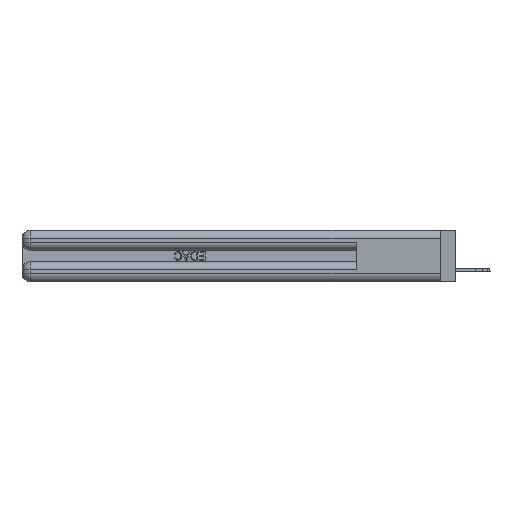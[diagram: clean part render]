
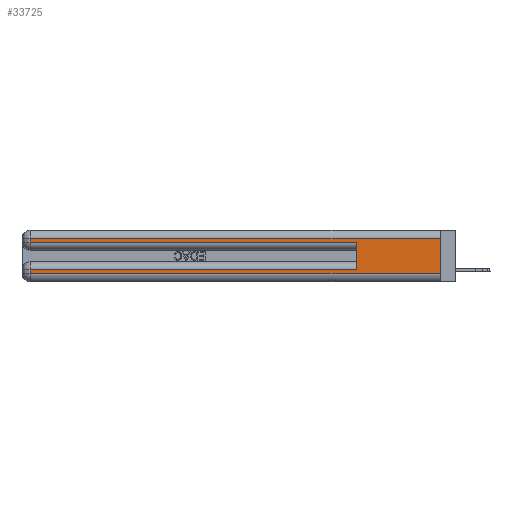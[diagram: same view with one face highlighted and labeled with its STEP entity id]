
A CAD part, left-side view. The second image highlights one B-rep face of the part: STEP entity #33725.
In plain terms, the highlighted planar face has unit normal (-1, 0, 0).
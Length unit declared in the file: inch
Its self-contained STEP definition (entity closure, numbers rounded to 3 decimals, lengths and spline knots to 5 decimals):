
#102 = DIRECTION ( 'NONE',  ( 0., -1., 0. ) ) ;
#220 = CARTESIAN_POINT ( 'NONE',  ( 0., 0., 0.285 ) ) ;
#392 = LINE ( 'NONE', #25619, #35999 ) ;
#620 = DIRECTION ( 'NONE',  ( 0., 1., 0. ) ) ;
#663 = EDGE_CURVE ( 'NONE', #34133, #27485, #3351, .T. ) ;
#842 = DIRECTION ( 'NONE',  ( 0., 0., -1. ) ) ;
#1767 = CARTESIAN_POINT ( 'NONE',  ( 0., 2.94, 0.285 ) ) ;
#1819 = CARTESIAN_POINT ( 'NONE',  ( 0., 0.6, 0.145 ) ) ;
#3016 = VERTEX_POINT ( 'NONE', #15526 ) ;
#3038 = VECTOR ( 'NONE', #6035, 39.37008 ) ;
#3351 = LINE ( 'NONE', #220, #6422 ) ;
#3595 = EDGE_CURVE ( 'NONE', #3016, #16636, #392, .T. ) ;
#4185 = LINE ( 'NONE', #19852, #24195 ) ;
#4633 = EDGE_LOOP ( 'NONE', ( #14149, #35008, #35609, #28040, #35874, #6933, #33448, #26361 ) ) ;
#5358 = AXIS2_PLACEMENT_3D ( 'NONE', #8840, #5862, #34517 ) ;
#5862 = DIRECTION ( 'NONE',  ( 1., 0., 0. ) ) ;
#6035 = DIRECTION ( 'NONE',  ( 0., 1., 0. ) ) ;
#6422 = VECTOR ( 'NONE', #20336, 39.37008 ) ;
#6619 = EDGE_CURVE ( 'NONE', #3016, #26334, #10309, .T. ) ;
#6933 = ORIENTED_EDGE ( 'NONE', *, *, #26800, .T. ) ;
#7056 = CARTESIAN_POINT ( 'NONE',  ( 0., 2.94, 0.31 ) ) ;
#8618 = DIRECTION ( 'NONE',  ( 0., 0., -1. ) ) ;
#8840 = CARTESIAN_POINT ( 'NONE',  ( 0., 0., 0.37 ) ) ;
#9144 = CARTESIAN_POINT ( 'NONE',  ( 0., 0., 0.31 ) ) ;
#9333 = CARTESIAN_POINT ( 'NONE',  ( 0., 2.94, 0.085 ) ) ;
#9844 = LINE ( 'NONE', #14206, #27217 ) ;
#10309 = LINE ( 'NONE', #9144, #31231 ) ;
#11201 = PLANE ( 'NONE',  #5358 ) ;
#14149 = ORIENTED_EDGE ( 'NONE', *, *, #3595, .F. ) ;
#14206 = CARTESIAN_POINT ( 'NONE',  ( 0., 2.94, 0.37 ) ) ;
#15469 = LINE ( 'NONE', #25588, #3038 ) ;
#15526 = CARTESIAN_POINT ( 'NONE',  ( 0., 0., 0.31 ) ) ;
#16636 = VERTEX_POINT ( 'NONE', #27970 ) ;
#16673 = VECTOR ( 'NONE', #27039, 39.37008 ) ;
#17575 = LINE ( 'NONE', #1819, #16673 ) ;
#18071 = CARTESIAN_POINT ( 'NONE',  ( 0., 2.94, 0.06 ) ) ;
#18139 = VERTEX_POINT ( 'NONE', #18071 ) ;
#18262 = CARTESIAN_POINT ( 'NONE',  ( 0., 0.6, 0.285 ) ) ;
#19852 = CARTESIAN_POINT ( 'NONE',  ( 0., 0., 0.06 ) ) ;
#20336 = DIRECTION ( 'NONE',  ( 0., -1., 0. ) ) ;
#20793 = EDGE_CURVE ( 'NONE', #26334, #34133, #9844, .T. ) ;
#21460 = FACE_OUTER_BOUND ( 'NONE', #4633, .T. ) ;
#24195 = VECTOR ( 'NONE', #102, 39.37008 ) ;
#25250 = EDGE_CURVE ( 'NONE', #29769, #27485, #17575, .T. ) ;
#25588 = CARTESIAN_POINT ( 'NONE',  ( 0., 0., 0.085 ) ) ;
#25619 = CARTESIAN_POINT ( 'NONE',  ( 0., 0., 0.37 ) ) ;
#25742 = VERTEX_POINT ( 'NONE', #9333 ) ;
#26334 = VERTEX_POINT ( 'NONE', #7056 ) ;
#26361 = ORIENTED_EDGE ( 'NONE', *, *, #32756, .T. ) ;
#26800 = EDGE_CURVE ( 'NONE', #29769, #25742, #15469, .T. ) ;
#27039 = DIRECTION ( 'NONE',  ( 0., 0., 1. ) ) ;
#27217 = VECTOR ( 'NONE', #8618, 39.37008 ) ;
#27485 = VERTEX_POINT ( 'NONE', #18262 ) ;
#27970 = CARTESIAN_POINT ( 'NONE',  ( 0., 0., 0.06 ) ) ;
#28040 = ORIENTED_EDGE ( 'NONE', *, *, #663, .T. ) ;
#28047 = EDGE_CURVE ( 'NONE', #25742, #18139, #36778, .T. ) ;
#28285 = VECTOR ( 'NONE', #842, 39.37008 ) ;
#28464 = DIRECTION ( 'NONE',  ( 0., 0., -1. ) ) ;
#29769 = VERTEX_POINT ( 'NONE', #32164 ) ;
#29770 = CARTESIAN_POINT ( 'NONE',  ( 0., 2.94, 0.37 ) ) ;
#31231 = VECTOR ( 'NONE', #620, 39.37008 ) ;
#32164 = CARTESIAN_POINT ( 'NONE',  ( 0., 0.6, 0.085 ) ) ;
#32756 = EDGE_CURVE ( 'NONE', #18139, #16636, #4185, .T. ) ;
#33448 = ORIENTED_EDGE ( 'NONE', *, *, #28047, .T. ) ;
#33725 = ADVANCED_FACE ( 'NONE', ( #21460 ), #11201, .F. ) ;
#34133 = VERTEX_POINT ( 'NONE', #1767 ) ;
#34517 = DIRECTION ( 'NONE',  ( 0., 0., -1. ) ) ;
#35008 = ORIENTED_EDGE ( 'NONE', *, *, #6619, .T. ) ;
#35609 = ORIENTED_EDGE ( 'NONE', *, *, #20793, .T. ) ;
#35874 = ORIENTED_EDGE ( 'NONE', *, *, #25250, .F. ) ;
#35999 = VECTOR ( 'NONE', #28464, 39.37008 ) ;
#36778 = LINE ( 'NONE', #29770, #28285 ) ;
